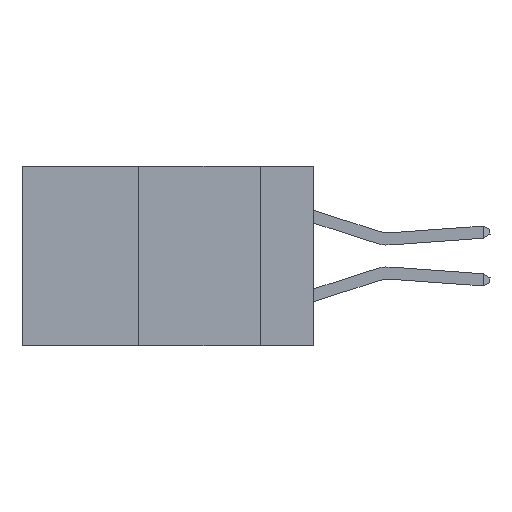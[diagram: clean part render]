
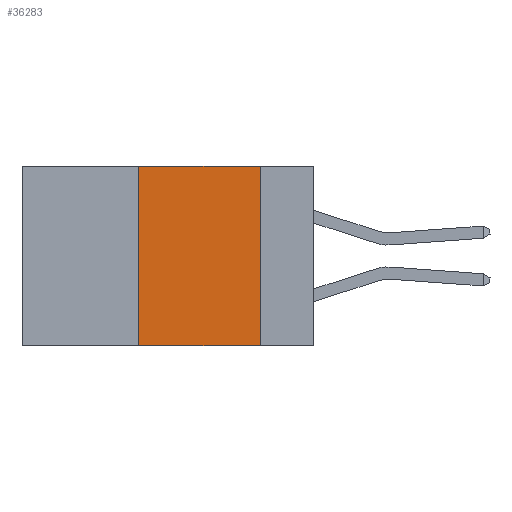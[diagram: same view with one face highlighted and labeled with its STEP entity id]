
A CAD part, left-side view. The second image highlights one B-rep face of the part: STEP entity #36283.
In plain terms, the highlighted planar face has unit normal (-1, 0, 0).
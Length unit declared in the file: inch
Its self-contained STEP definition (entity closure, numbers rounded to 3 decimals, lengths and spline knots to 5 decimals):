
#1126 = CARTESIAN_POINT ( 'NONE',  ( 0., 0.6, 0. ) ) ;
#2030 = AXIS2_PLACEMENT_3D ( 'NONE', #11524, #33269, #14708 ) ;
#3057 = LINE ( 'NONE', #14042, #18839 ) ;
#3329 = LINE ( 'NONE', #26079, #26333 ) ;
#3501 = VECTOR ( 'NONE', #39623, 39.37008 ) ;
#4325 = DIRECTION ( 'NONE',  ( 0., -1., 0. ) ) ;
#6565 = EDGE_CURVE ( 'NONE', #30027, #19243, #3057, .T. ) ;
#9765 = ORIENTED_EDGE ( 'NONE', *, *, #33966, .F. ) ;
#11524 = CARTESIAN_POINT ( 'NONE',  ( 0., 0.6, 0. ) ) ;
#14042 = CARTESIAN_POINT ( 'NONE',  ( 0., 0.36, 0. ) ) ;
#14360 = VECTOR ( 'NONE', #4325, 39.37008 ) ;
#14708 = DIRECTION ( 'NONE',  ( 0., 0., -1. ) ) ;
#14817 = EDGE_CURVE ( 'NONE', #30027, #31229, #3329, .T. ) ;
#16033 = EDGE_LOOP ( 'NONE', ( #9765, #29632, #37947, #22971 ) ) ;
#16889 = CARTESIAN_POINT ( 'NONE',  ( 0., 0.11, 0. ) ) ;
#18254 = CARTESIAN_POINT ( 'NONE',  ( 0., 0.11, -0.37 ) ) ;
#18839 = VECTOR ( 'NONE', #29475, 39.37008 ) ;
#19243 = VERTEX_POINT ( 'NONE', #34388 ) ;
#19472 = VERTEX_POINT ( 'NONE', #16889 ) ;
#20807 = PLANE ( 'NONE',  #2030 ) ;
#22971 = ORIENTED_EDGE ( 'NONE', *, *, #14817, .T. ) ;
#24494 = FACE_OUTER_BOUND ( 'NONE', #16033, .T. ) ;
#25350 = EDGE_CURVE ( 'NONE', #19243, #19472, #39033, .T. ) ;
#26079 = CARTESIAN_POINT ( 'NONE',  ( 0., 0.6, -0.37 ) ) ;
#26333 = VECTOR ( 'NONE', #29191, 39.37008 ) ;
#28336 = CARTESIAN_POINT ( 'NONE',  ( 0., 0.36, -0.37 ) ) ;
#28449 = LINE ( 'NONE', #36568, #3501 ) ;
#29191 = DIRECTION ( 'NONE',  ( 0., -1., 0. ) ) ;
#29475 = DIRECTION ( 'NONE',  ( 0., 0., 1. ) ) ;
#29632 = ORIENTED_EDGE ( 'NONE', *, *, #25350, .F. ) ;
#30027 = VERTEX_POINT ( 'NONE', #28336 ) ;
#31229 = VERTEX_POINT ( 'NONE', #18254 ) ;
#33269 = DIRECTION ( 'NONE',  ( 1., 0., 0. ) ) ;
#33966 = EDGE_CURVE ( 'NONE', #19472, #31229, #28449, .T. ) ;
#34388 = CARTESIAN_POINT ( 'NONE',  ( 0., 0.36, 0. ) ) ;
#36283 = ADVANCED_FACE ( 'NONE', ( #24494 ), #20807, .F. ) ;
#36568 = CARTESIAN_POINT ( 'NONE',  ( 0., 0.11, 0. ) ) ;
#37947 = ORIENTED_EDGE ( 'NONE', *, *, #6565, .F. ) ;
#39033 = LINE ( 'NONE', #1126, #14360 ) ;
#39623 = DIRECTION ( 'NONE',  ( 0., 0., -1. ) ) ;
